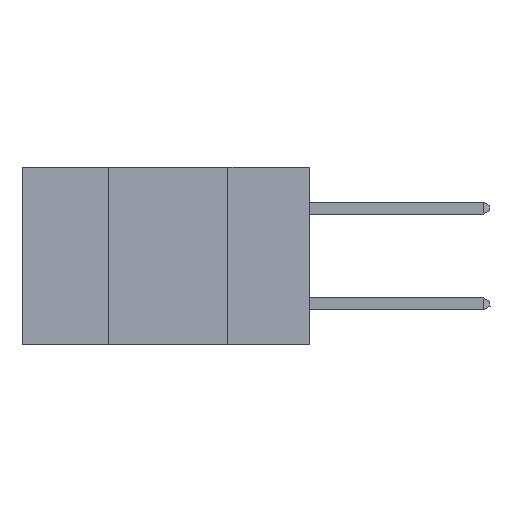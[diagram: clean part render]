
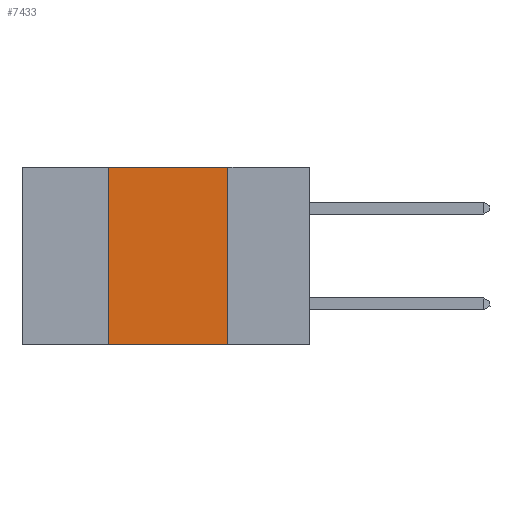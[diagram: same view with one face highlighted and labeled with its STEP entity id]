
A CAD part, left-side view. The second image highlights one B-rep face of the part: STEP entity #7433.
In plain terms, the highlighted planar face has unit normal (-1, 0, 0).
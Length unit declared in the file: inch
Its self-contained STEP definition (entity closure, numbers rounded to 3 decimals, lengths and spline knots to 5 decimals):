
#446 = VERTEX_POINT ( 'NONE', #15219 ) ;
#704 = LINE ( 'NONE', #18719, #18868 ) ;
#1014 = DIRECTION ( 'NONE',  ( 0., -1., 0. ) ) ;
#1239 = VERTEX_POINT ( 'NONE', #16131 ) ;
#1794 = CARTESIAN_POINT ( 'NONE',  ( 0., 0.6, 0. ) ) ;
#4290 = CARTESIAN_POINT ( 'NONE',  ( 0., 0.42, 0. ) ) ;
#4771 = CARTESIAN_POINT ( 'NONE',  ( 0., 0.6, -0.37 ) ) ;
#5022 = EDGE_LOOP ( 'NONE', ( #15127, #12201, #20046, #22408 ) ) ;
#5035 = EDGE_CURVE ( 'NONE', #1239, #9017, #19279, .T. ) ;
#5576 = CARTESIAN_POINT ( 'NONE',  ( 0., 0.17, -0.37 ) ) ;
#5697 = VERTEX_POINT ( 'NONE', #4290 ) ;
#7433 = ADVANCED_FACE ( 'NONE', ( #13440 ), #14971, .F. ) ;
#7459 = DIRECTION ( 'NONE',  ( 0., -1., 0. ) ) ;
#8886 = EDGE_CURVE ( 'NONE', #446, #5697, #704, .T. ) ;
#9017 = VERTEX_POINT ( 'NONE', #5576 ) ;
#9830 = DIRECTION ( 'NONE',  ( 0., 0., -1. ) ) ;
#10974 = VECTOR ( 'NONE', #7459, 39.37008 ) ;
#12201 = ORIENTED_EDGE ( 'NONE', *, *, #15956, .F. ) ;
#12858 = EDGE_CURVE ( 'NONE', #446, #9017, #15955, .T. ) ;
#13440 = FACE_OUTER_BOUND ( 'NONE', #5022, .T. ) ;
#14873 = VECTOR ( 'NONE', #21317, 39.37008 ) ;
#14893 = VECTOR ( 'NONE', #1014, 39.37008 ) ;
#14971 = PLANE ( 'NONE',  #20730 ) ;
#15127 = ORIENTED_EDGE ( 'NONE', *, *, #5035, .F. ) ;
#15219 = CARTESIAN_POINT ( 'NONE',  ( 0., 0.42, -0.37 ) ) ;
#15448 = DIRECTION ( 'NONE',  ( 0., 0., 1. ) ) ;
#15955 = LINE ( 'NONE', #4771, #14893 ) ;
#15956 = EDGE_CURVE ( 'NONE', #5697, #1239, #19919, .T. ) ;
#16131 = CARTESIAN_POINT ( 'NONE',  ( 0., 0.17, 0. ) ) ;
#16697 = CARTESIAN_POINT ( 'NONE',  ( 0., 0.6, 0. ) ) ;
#18719 = CARTESIAN_POINT ( 'NONE',  ( 0., 0.42, 0. ) ) ;
#18868 = VECTOR ( 'NONE', #15448, 39.37008 ) ;
#19279 = LINE ( 'NONE', #21412, #14873 ) ;
#19919 = LINE ( 'NONE', #1794, #10974 ) ;
#19968 = DIRECTION ( 'NONE',  ( 1., 0., 0. ) ) ;
#20046 = ORIENTED_EDGE ( 'NONE', *, *, #8886, .F. ) ;
#20730 = AXIS2_PLACEMENT_3D ( 'NONE', #16697, #19968, #9830 ) ;
#21317 = DIRECTION ( 'NONE',  ( 0., 0., -1. ) ) ;
#21412 = CARTESIAN_POINT ( 'NONE',  ( 0., 0.17, 0. ) ) ;
#22408 = ORIENTED_EDGE ( 'NONE', *, *, #12858, .T. ) ;
